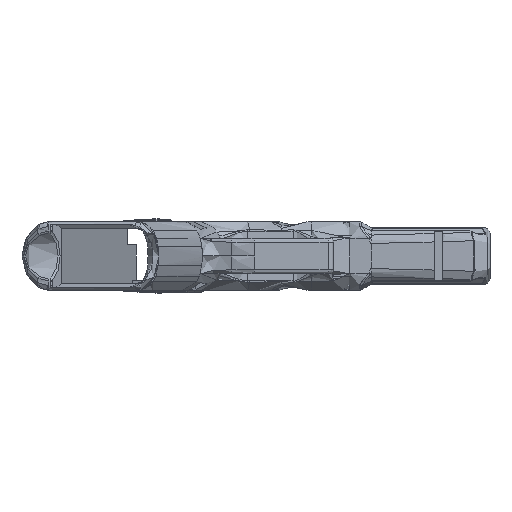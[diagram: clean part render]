
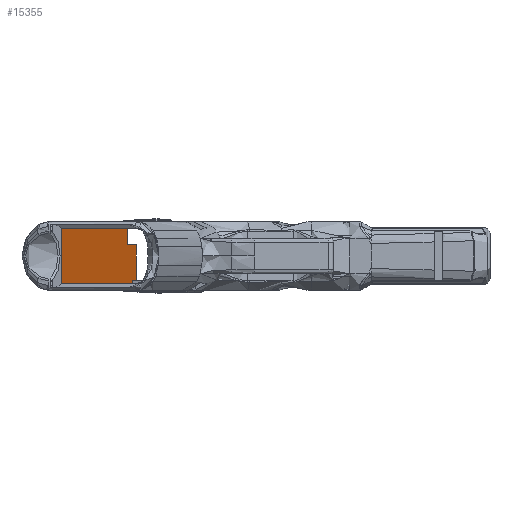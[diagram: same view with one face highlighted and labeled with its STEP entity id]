
A CAD part, front view. The second image highlights one B-rep face of the part: STEP entity #15355.
In plain terms, the highlighted planar face has unit normal (0.951, -0.309, 0).
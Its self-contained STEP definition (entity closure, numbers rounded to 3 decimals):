
#1311=ELLIPSE('',#15856,1.051,1.);
#1320=ELLIPSE('',#15881,1.051,1.);
#2778=FACE_OUTER_BOUND('',#3678,.T.);
#3678=EDGE_LOOP('',(#13095,#13096,#13097,#13098,#13099,#13100,#13101,#13102,
#13103,#13104));
#4188=LINE('',#21339,#5111);
#4210=LINE('',#21794,#5133);
#4221=LINE('',#22108,#5144);
#4609=LINE('',#42701,#5532);
#4700=LINE('',#49385,#5623);
#4702=LINE('',#49871,#5625);
#4724=LINE('',#51703,#5647);
#4725=LINE('',#51704,#5648);
#5111=VECTOR('',#17507,10.);
#5133=VECTOR('',#17551,10.);
#5144=VECTOR('',#17588,10.);
#5532=VECTOR('',#19000,10.);
#5623=VECTOR('',#19343,10.);
#5625=VECTOR('',#19349,10.);
#5647=VECTOR('',#19427,10.);
#5648=VECTOR('',#19428,10.);
#6014=VERTEX_POINT('',#20784);
#6015=VERTEX_POINT('',#20785);
#6046=VERTEX_POINT('',#21338);
#6067=VERTEX_POINT('',#21766);
#6069=VERTEX_POINT('',#21770);
#6079=VERTEX_POINT('',#21792);
#6851=VERTEX_POINT('',#42699);
#6992=VERTEX_POINT('',#49384);
#6998=VERTEX_POINT('',#49869);
#6999=VERTEX_POINT('',#49870);
#7640=EDGE_CURVE('',#6014,#6015,#1311,.F.);
#7681=EDGE_CURVE('',#6046,#6015,#4188,.T.);
#7711=EDGE_CURVE('',#6069,#6067,#1320,.F.);
#7722=EDGE_CURVE('',#6069,#6079,#4210,.T.);
#7752=EDGE_CURVE('',#6067,#6014,#4221,.F.);
#8867=EDGE_CURVE('',#6851,#6079,#4609,.T.);
#9103=EDGE_CURVE('',#6992,#6851,#4700,.T.);
#9112=EDGE_CURVE('',#6998,#6999,#4702,.T.);
#9178=EDGE_CURVE('',#6999,#6992,#4724,.T.);
#9179=EDGE_CURVE('',#6046,#6998,#4725,.T.);
#13095=ORIENTED_EDGE('',*,*,#7681,.T.);
#13096=ORIENTED_EDGE('',*,*,#7640,.F.);
#13097=ORIENTED_EDGE('',*,*,#7752,.F.);
#13098=ORIENTED_EDGE('',*,*,#7711,.F.);
#13099=ORIENTED_EDGE('',*,*,#7722,.T.);
#13100=ORIENTED_EDGE('',*,*,#8867,.F.);
#13101=ORIENTED_EDGE('',*,*,#9103,.F.);
#13102=ORIENTED_EDGE('',*,*,#9178,.F.);
#13103=ORIENTED_EDGE('',*,*,#9112,.F.);
#13104=ORIENTED_EDGE('',*,*,#9179,.F.);
#14678=PLANE('',#16563);
#15355=ADVANCED_FACE('',(#2778),#14678,.F.);
#15856=AXIS2_PLACEMENT_3D('',#20786,#17469,#17470);
#15881=AXIS2_PLACEMENT_3D('',#21772,#17537,#17538);
#16563=AXIS2_PLACEMENT_3D('',#51702,#19425,#19426);
#17469=DIRECTION('center_axis',(-0.951,0.309,0.));
#17470=DIRECTION('ref_axis',(-0.309,-0.951,0.));
#17507=DIRECTION('',(-0.309,-0.951,0.));
#17537=DIRECTION('center_axis',(-0.951,0.309,0.));
#17538=DIRECTION('ref_axis',(-0.309,-0.951,0.));
#17551=DIRECTION('',(0.309,0.951,0.));
#17588=DIRECTION('',(0.,0.,-1.));
#19000=DIRECTION('',(0.,0.,-1.));
#19343=DIRECTION('',(-0.309,-0.951,0.));
#19349=DIRECTION('',(0.309,0.951,0.));
#19425=DIRECTION('center_axis',(-0.951,0.309,0.));
#19426=DIRECTION('ref_axis',(0.,0.,
1.));
#19427=DIRECTION('',(0.,0.,-1.));
#19428=DIRECTION('',(0.,0.,-1.));
#20784=CARTESIAN_POINT('',(2.236,-98.,11.766));
#20785=CARTESIAN_POINT('',(2.294,-97.822,11.75));
#20786=CARTESIAN_POINT('Origin',(2.294,-97.822,12.75));
#21338=CARTESIAN_POINT('',(30.049,-12.4,11.75));
#21339=CARTESIAN_POINT('',(2.312,-97.765,11.75));
#21766=CARTESIAN_POINT('',(2.236,-98.,-11.766));
#21770=CARTESIAN_POINT('',(2.294,-97.822,-11.75));
#21772=CARTESIAN_POINT('Origin',(2.294,-97.822,-12.75));
#21792=CARTESIAN_POINT('',(32.169,-5.875,-11.75));
#21794=CARTESIAN_POINT('',(2.312,-97.765,-11.75));
#22108=CARTESIAN_POINT('',(2.236,-98.,-18.375));
#42699=CARTESIAN_POINT('',(32.169,-5.875,-10.375));
#42701=CARTESIAN_POINT('',(32.169,-5.875,-5.875));
#49384=CARTESIAN_POINT('',(33.591,-1.5,-10.375));
#49385=CARTESIAN_POINT('',(17.241,-51.82,-10.375));
#49869=CARTESIAN_POINT('',(30.049,-12.4,4.75));
#49870=CARTESIAN_POINT('',(33.591,-1.5,4.75));
#49871=CARTESIAN_POINT('',(18.86,-46.836,4.75));
#51702=CARTESIAN_POINT('Origin',(2.312,-97.765,-11.75));
#51703=CARTESIAN_POINT('',(33.591,-1.5,-5.875));
#51704=CARTESIAN_POINT('',(30.049,-12.4,2.982));
